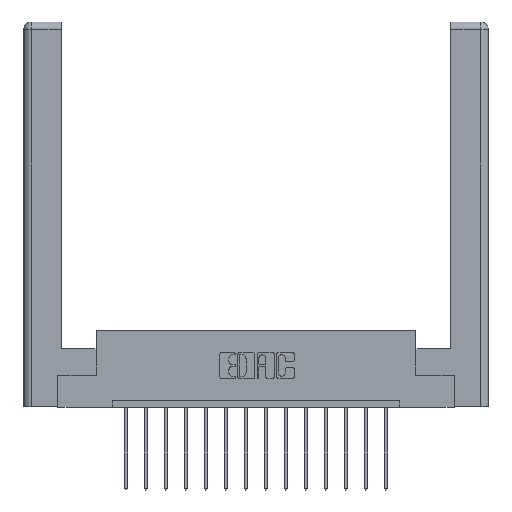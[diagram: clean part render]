
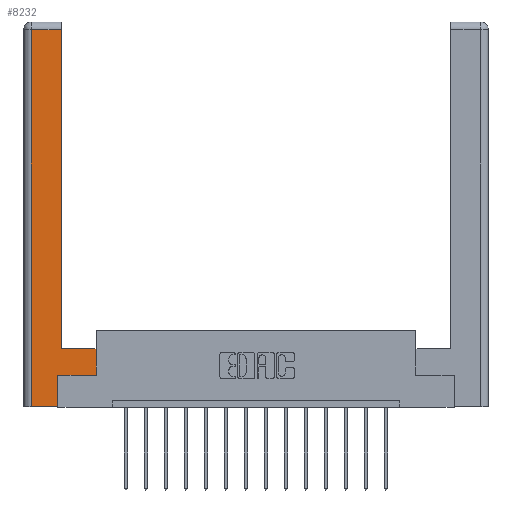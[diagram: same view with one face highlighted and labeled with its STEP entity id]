
A CAD part, top view. The second image highlights one B-rep face of the part: STEP entity #8232.
In plain terms, the highlighted planar face has unit normal (0, 0, 1).
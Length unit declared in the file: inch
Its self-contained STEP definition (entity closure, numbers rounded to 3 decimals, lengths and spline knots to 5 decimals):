
#23 = VECTOR ( 'NONE', #7482, 39.37008 ) ;
#112 = CARTESIAN_POINT ( 'NONE',  ( 0.295, 0.45, 0. ) ) ;
#290 = VECTOR ( 'NONE', #12327, 39.37008 ) ;
#541 = DIRECTION ( 'NONE',  ( 0., 1., 0. ) ) ;
#560 = ORIENTED_EDGE ( 'NONE', *, *, #12385, .T. ) ;
#779 = PLANE ( 'NONE',  #4867 ) ;
#1082 = CARTESIAN_POINT ( 'NONE',  ( 0.565, 0.245, 0. ) ) ;
#1197 = ORIENTED_EDGE ( 'NONE', *, *, #10298, .T. ) ;
#1294 = VECTOR ( 'NONE', #6867, 39.37008 ) ;
#1327 = DIRECTION ( 'NONE',  ( 0., -1., 0. ) ) ;
#1487 = LINE ( 'NONE', #13099, #1294 ) ;
#1811 = VERTEX_POINT ( 'NONE', #4151 ) ;
#2159 = DIRECTION ( 'NONE',  ( 1., 0., 0. ) ) ;
#2369 = EDGE_CURVE ( 'NONE', #13752, #11526, #12222, .T. ) ;
#2381 = VECTOR ( 'NONE', #1327, 39.37008 ) ;
#2569 = CARTESIAN_POINT ( 'NONE',  ( 0.265, 0., 0. ) ) ;
#2995 = VECTOR ( 'NONE', #4074, 39.37008 ) ;
#3200 = CARTESIAN_POINT ( 'NONE',  ( 0.0615, 2.94, 0. ) ) ;
#4074 = DIRECTION ( 'NONE',  ( -1., 0., 0. ) ) ;
#4151 = CARTESIAN_POINT ( 'NONE',  ( 0.565, 0.245, 0. ) ) ;
#4301 = CARTESIAN_POINT ( 'NONE',  ( 0.295, 3., 0. ) ) ;
#4867 = AXIS2_PLACEMENT_3D ( 'NONE', #8822, #11521, #12583 ) ;
#5047 = EDGE_CURVE ( 'NONE', #9202, #5137, #9450, .T. ) ;
#5051 = ORIENTED_EDGE ( 'NONE', *, *, #10835, .T. ) ;
#5137 = VERTEX_POINT ( 'NONE', #9032 ) ;
#5341 = VECTOR ( 'NONE', #2159, 39.37008 ) ;
#5816 = LINE ( 'NONE', #12828, #2381 ) ;
#6176 = LINE ( 'NONE', #15129, #290 ) ;
#6867 = DIRECTION ( 'NONE',  ( 0., 1., 0. ) ) ;
#7367 = EDGE_CURVE ( 'NONE', #1811, #15040, #1487, .T. ) ;
#7482 = DIRECTION ( 'NONE',  ( 1., 0., 0. ) ) ;
#8073 = ORIENTED_EDGE ( 'NONE', *, *, #5047, .T. ) ;
#8232 = ADVANCED_FACE ( 'NONE', ( #8945 ), #779, .F. ) ;
#8602 = CARTESIAN_POINT ( 'NONE',  ( 0.0615, 0., 0. ) ) ;
#8679 = VECTOR ( 'NONE', #541, 39.37008 ) ;
#8822 = CARTESIAN_POINT ( 'NONE',  ( 0., 0., 0. ) ) ;
#8945 = FACE_OUTER_BOUND ( 'NONE', #14450, .T. ) ;
#9032 = CARTESIAN_POINT ( 'NONE',  ( 0.295, 2.94, 0. ) ) ;
#9202 = VERTEX_POINT ( 'NONE', #112 ) ;
#9450 = LINE ( 'NONE', #4301, #8679 ) ;
#9566 = DIRECTION ( 'NONE',  ( -1., 0., 0. ) ) ;
#10298 = EDGE_CURVE ( 'NONE', #15040, #9202, #16507, .T. ) ;
#10776 = VERTEX_POINT ( 'NONE', #12693 ) ;
#10835 = EDGE_CURVE ( 'NONE', #5137, #14456, #14449, .T. ) ;
#10979 = ORIENTED_EDGE ( 'NONE', *, *, #14471, .T. ) ;
#11263 = CARTESIAN_POINT ( 'NONE',  ( 0.265, 0., 0. ) ) ;
#11487 = EDGE_CURVE ( 'NONE', #14456, #13752, #5816, .T. ) ;
#11521 = DIRECTION ( 'NONE',  ( 0., 0., -1. ) ) ;
#11526 = VERTEX_POINT ( 'NONE', #2569 ) ;
#11558 = ORIENTED_EDGE ( 'NONE', *, *, #2369, .T. ) ;
#11567 = CARTESIAN_POINT ( 'NONE',  ( 0.565, 0.45, 0. ) ) ;
#12028 = CARTESIAN_POINT ( 'NONE',  ( 0.0615, 2.94, 0. ) ) ;
#12222 = LINE ( 'NONE', #11263, #5341 ) ;
#12327 = DIRECTION ( 'NONE',  ( 0., 1., 0. ) ) ;
#12385 = EDGE_CURVE ( 'NONE', #11526, #10776, #6176, .T. ) ;
#12583 = DIRECTION ( 'NONE',  ( -1., 0., 0. ) ) ;
#12693 = CARTESIAN_POINT ( 'NONE',  ( 0.265, 0.245, 0. ) ) ;
#12828 = CARTESIAN_POINT ( 'NONE',  ( 0.0615, 0., 0. ) ) ;
#12934 = LINE ( 'NONE', #1082, #23 ) ;
#13099 = CARTESIAN_POINT ( 'NONE',  ( 0.565, 0.45, 0. ) ) ;
#13487 = VECTOR ( 'NONE', #9566, 39.37008 ) ;
#13752 = VERTEX_POINT ( 'NONE', #8602 ) ;
#14449 = LINE ( 'NONE', #3200, #13487 ) ;
#14450 = EDGE_LOOP ( 'NONE', ( #8073, #5051, #15028, #11558, #560, #10979, #15905, #1197 ) ) ;
#14456 = VERTEX_POINT ( 'NONE', #12028 ) ;
#14471 = EDGE_CURVE ( 'NONE', #10776, #1811, #12934, .T. ) ;
#14524 = CARTESIAN_POINT ( 'NONE',  ( 0.295, 0.45, 0. ) ) ;
#15028 = ORIENTED_EDGE ( 'NONE', *, *, #11487, .T. ) ;
#15040 = VERTEX_POINT ( 'NONE', #11567 ) ;
#15129 = CARTESIAN_POINT ( 'NONE',  ( 0.265, 0.245, 0. ) ) ;
#15905 = ORIENTED_EDGE ( 'NONE', *, *, #7367, .T. ) ;
#16507 = LINE ( 'NONE', #14524, #2995 ) ;
